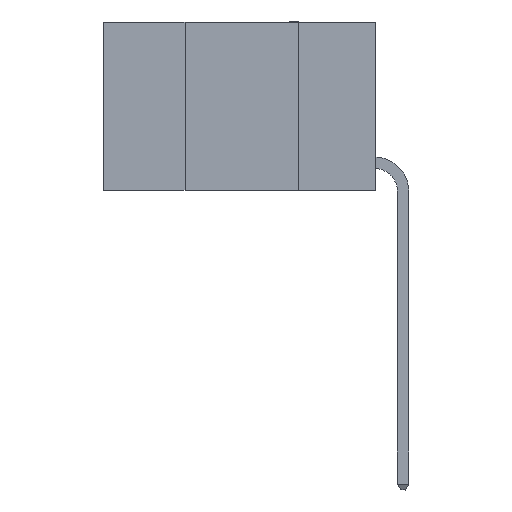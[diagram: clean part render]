
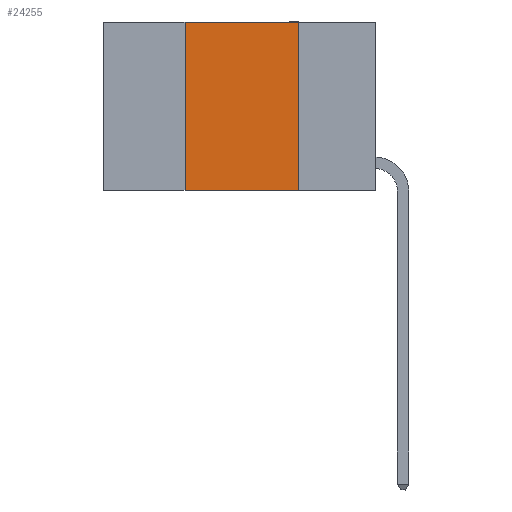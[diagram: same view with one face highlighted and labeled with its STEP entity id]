
A CAD part, left-side view. The second image highlights one B-rep face of the part: STEP entity #24255.
In plain terms, the highlighted planar face has unit normal (-1, 0, 0).
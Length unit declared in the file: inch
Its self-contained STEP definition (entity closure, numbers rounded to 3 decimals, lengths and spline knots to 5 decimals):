
#75 = DIRECTION ( 'NONE',  ( 0., -1., 0. ) ) ;
#1088 = EDGE_LOOP ( 'NONE', ( #15683, #5096, #14842, #15660 ) ) ;
#1640 = VECTOR ( 'NONE', #7785, 39.37008 ) ;
#1722 = LINE ( 'NONE', #7281, #19983 ) ;
#2148 = CARTESIAN_POINT ( 'NONE',  ( 0., 0.42, 0. ) ) ;
#4462 = AXIS2_PLACEMENT_3D ( 'NONE', #17980, #8232, #16051 ) ;
#5096 = ORIENTED_EDGE ( 'NONE', *, *, #8328, .F. ) ;
#5121 = VERTEX_POINT ( 'NONE', #9545 ) ;
#5370 = CARTESIAN_POINT ( 'NONE',  ( 0., 0.6, 0. ) ) ;
#6614 = VERTEX_POINT ( 'NONE', #17553 ) ;
#7135 = EDGE_CURVE ( 'NONE', #5121, #22931, #21865, .T. ) ;
#7281 = CARTESIAN_POINT ( 'NONE',  ( 0., 0.17, 0. ) ) ;
#7779 = CARTESIAN_POINT ( 'NONE',  ( 0., 0.6, -0.37 ) ) ;
#7785 = DIRECTION ( 'NONE',  ( 0., -1., 0. ) ) ;
#8232 = DIRECTION ( 'NONE',  ( 1., 0., 0. ) ) ;
#8328 = EDGE_CURVE ( 'NONE', #10404, #6614, #24844, .T. ) ;
#9545 = CARTESIAN_POINT ( 'NONE',  ( 0., 0.42, -0.37 ) ) ;
#10024 = FACE_OUTER_BOUND ( 'NONE', #1088, .T. ) ;
#10404 = VERTEX_POINT ( 'NONE', #22827 ) ;
#13593 = DIRECTION ( 'NONE',  ( 0., 0., 1. ) ) ;
#13796 = VECTOR ( 'NONE', #75, 39.37008 ) ;
#14842 = ORIENTED_EDGE ( 'NONE', *, *, #16085, .F. ) ;
#15279 = VECTOR ( 'NONE', #13593, 39.37008 ) ;
#15660 = ORIENTED_EDGE ( 'NONE', *, *, #7135, .T. ) ;
#15683 = ORIENTED_EDGE ( 'NONE', *, *, #23523, .F. ) ;
#16051 = DIRECTION ( 'NONE',  ( 0., 0., -1. ) ) ;
#16085 = EDGE_CURVE ( 'NONE', #5121, #10404, #19734, .T. ) ;
#17553 = CARTESIAN_POINT ( 'NONE',  ( 0., 0.17, 0. ) ) ;
#17848 = PLANE ( 'NONE',  #4462 ) ;
#17980 = CARTESIAN_POINT ( 'NONE',  ( 0., 0.6, 0. ) ) ;
#19734 = LINE ( 'NONE', #2148, #15279 ) ;
#19983 = VECTOR ( 'NONE', #23024, 39.37008 ) ;
#20250 = CARTESIAN_POINT ( 'NONE',  ( 0., 0.17, -0.37 ) ) ;
#21865 = LINE ( 'NONE', #7779, #13796 ) ;
#22827 = CARTESIAN_POINT ( 'NONE',  ( 0., 0.42, 0. ) ) ;
#22931 = VERTEX_POINT ( 'NONE', #20250 ) ;
#23024 = DIRECTION ( 'NONE',  ( 0., 0., -1. ) ) ;
#23523 = EDGE_CURVE ( 'NONE', #6614, #22931, #1722, .T. ) ;
#24255 = ADVANCED_FACE ( 'NONE', ( #10024 ), #17848, .F. ) ;
#24844 = LINE ( 'NONE', #5370, #1640 ) ;
